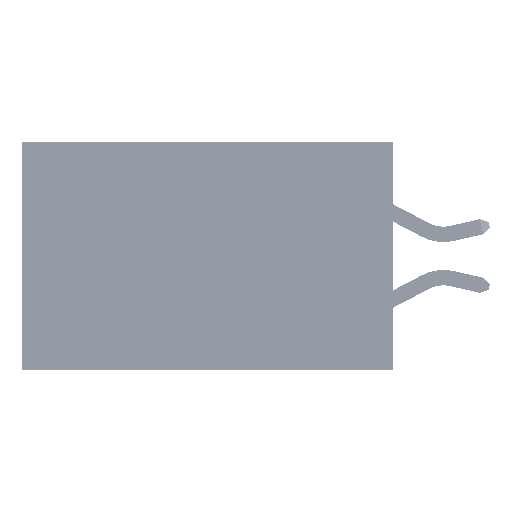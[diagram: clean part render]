
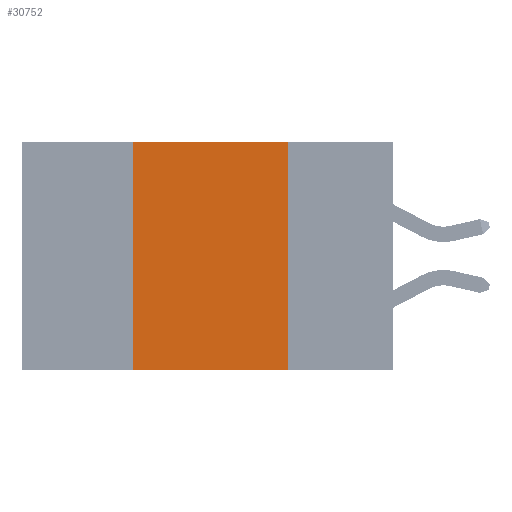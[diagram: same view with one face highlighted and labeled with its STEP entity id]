
A CAD part, left-side view. The second image highlights one B-rep face of the part: STEP entity #30752.
In plain terms, the highlighted planar face has unit normal (-1, 0, 0).
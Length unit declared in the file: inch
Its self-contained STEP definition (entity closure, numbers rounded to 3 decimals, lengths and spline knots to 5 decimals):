
#1799 = CARTESIAN_POINT ( 'NONE',  ( 0., 0.6, 0. ) ) ;
#1885 = CARTESIAN_POINT ( 'NONE',  ( 0., 0.17, -0.37 ) ) ;
#2343 = ORIENTED_EDGE ( 'NONE', *, *, #3890, .T. ) ;
#2442 = PLANE ( 'NONE',  #4592 ) ;
#3375 = CARTESIAN_POINT ( 'NONE',  ( 0., 0.42, 0. ) ) ;
#3890 = EDGE_CURVE ( 'NONE', #28938, #17475, #15909, .T. ) ;
#4136 = VECTOR ( 'NONE', #20346, 39.37008 ) ;
#4592 = AXIS2_PLACEMENT_3D ( 'NONE', #44633, #6191, #31193 ) ;
#6191 = DIRECTION ( 'NONE',  ( 1., 0., 0. ) ) ;
#7338 = EDGE_CURVE ( 'NONE', #8557, #17475, #30054, .T. ) ;
#7468 = EDGE_CURVE ( 'NONE', #39751, #8557, #33779, .T. ) ;
#8557 = VERTEX_POINT ( 'NONE', #24744 ) ;
#8833 = DIRECTION ( 'NONE',  ( 0., 0., -1. ) ) ;
#13353 = CARTESIAN_POINT ( 'NONE',  ( 0., 0.42, 0. ) ) ;
#14734 = VECTOR ( 'NONE', #41821, 39.37008 ) ;
#14780 = EDGE_CURVE ( 'NONE', #28938, #39751, #28421, .T. ) ;
#15909 = LINE ( 'NONE', #41343, #14734 ) ;
#17475 = VERTEX_POINT ( 'NONE', #1885 ) ;
#20346 = DIRECTION ( 'NONE',  ( 0., -1., 0. ) ) ;
#21836 = ORIENTED_EDGE ( 'NONE', *, *, #14780, .F. ) ;
#23183 = CARTESIAN_POINT ( 'NONE',  ( 0., 0.17, 0. ) ) ;
#24744 = CARTESIAN_POINT ( 'NONE',  ( 0., 0.17, 0. ) ) ;
#25823 = EDGE_LOOP ( 'NONE', ( #27210, #32042, #21836, #2343 ) ) ;
#27210 = ORIENTED_EDGE ( 'NONE', *, *, #7338, .F. ) ;
#28421 = LINE ( 'NONE', #3375, #38509 ) ;
#28605 = DIRECTION ( 'NONE',  ( 0., 0., 1. ) ) ;
#28938 = VERTEX_POINT ( 'NONE', #44922 ) ;
#30054 = LINE ( 'NONE', #23183, #36916 ) ;
#30752 = ADVANCED_FACE ( 'NONE', ( #33443 ), #2442, .F. ) ;
#31193 = DIRECTION ( 'NONE',  ( 0., 0., -1. ) ) ;
#32042 = ORIENTED_EDGE ( 'NONE', *, *, #7468, .F. ) ;
#33443 = FACE_OUTER_BOUND ( 'NONE', #25823, .T. ) ;
#33779 = LINE ( 'NONE', #1799, #4136 ) ;
#36916 = VECTOR ( 'NONE', #8833, 39.37008 ) ;
#38509 = VECTOR ( 'NONE', #28605, 39.37008 ) ;
#39751 = VERTEX_POINT ( 'NONE', #13353 ) ;
#41343 = CARTESIAN_POINT ( 'NONE',  ( 0., 0.6, -0.37 ) ) ;
#41821 = DIRECTION ( 'NONE',  ( 0., -1., 0. ) ) ;
#44633 = CARTESIAN_POINT ( 'NONE',  ( 0., 0.6, 0. ) ) ;
#44922 = CARTESIAN_POINT ( 'NONE',  ( 0., 0.42, -0.37 ) ) ;
